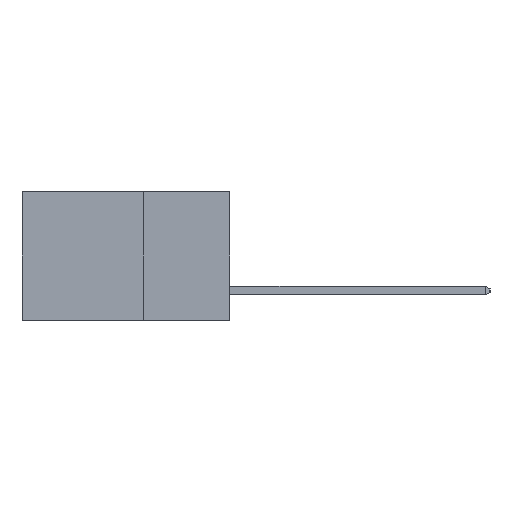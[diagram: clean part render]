
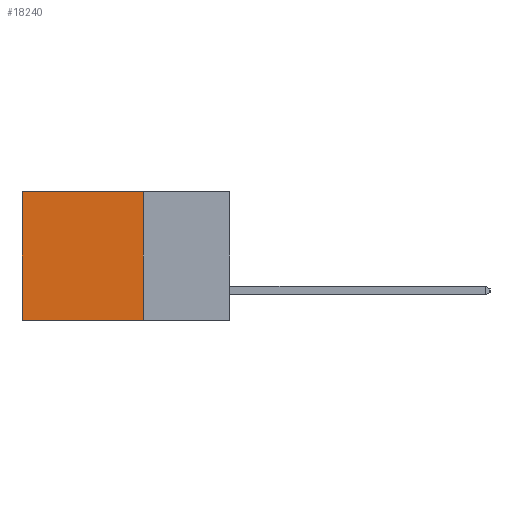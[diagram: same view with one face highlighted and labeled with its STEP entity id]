
A CAD part, left-side view. The second image highlights one B-rep face of the part: STEP entity #18240.
In plain terms, the highlighted planar face has unit normal (-1, 0, 0).
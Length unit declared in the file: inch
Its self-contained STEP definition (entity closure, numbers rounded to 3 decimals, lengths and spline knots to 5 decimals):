
#406 = VERTEX_POINT ( 'NONE', #3370 ) ;
#1237 = ORIENTED_EDGE ( 'NONE', *, *, #3281, .F. ) ;
#3281 = EDGE_CURVE ( 'NONE', #28011, #23730, #18194, .T. ) ;
#3370 = CARTESIAN_POINT ( 'NONE',  ( 0.298, 0.6, 0. ) ) ;
#4004 = CARTESIAN_POINT ( 'NONE',  ( 0.298, 0.6, -0.37 ) ) ;
#5310 = EDGE_CURVE ( 'NONE', #406, #12613, #32222, .T. ) ;
#5362 = VECTOR ( 'NONE', #13731, 39.37008 ) ;
#6385 = AXIS2_PLACEMENT_3D ( 'NONE', #22246, #7437, #24851 ) ;
#7437 = DIRECTION ( 'NONE',  ( 1., 0., 0. ) ) ;
#8690 = EDGE_LOOP ( 'NONE', ( #11857, #28076, #1237, #14813 ) ) ;
#8990 = CARTESIAN_POINT ( 'NONE',  ( 0.298, 0.6, 0. ) ) ;
#11723 = CARTESIAN_POINT ( 'NONE',  ( 0.298, 0.25, 0. ) ) ;
#11857 = ORIENTED_EDGE ( 'NONE', *, *, #5310, .T. ) ;
#12613 = VERTEX_POINT ( 'NONE', #4004 ) ;
#13731 = DIRECTION ( 'NONE',  ( 0., 1., 0. ) ) ;
#14813 = ORIENTED_EDGE ( 'NONE', *, *, #19359, .T. ) ;
#15311 = LINE ( 'NONE', #24009, #21906 ) ;
#17432 = VECTOR ( 'NONE', #25183, 39.37008 ) ;
#17674 = LINE ( 'NONE', #31253, #5362 ) ;
#18046 = VECTOR ( 'NONE', #29323, 39.37008 ) ;
#18194 = LINE ( 'NONE', #19132, #17432 ) ;
#18240 = ADVANCED_FACE ( 'NONE', ( #25203 ), #29758, .F. ) ;
#18876 = DIRECTION ( 'NONE',  ( 0., 1., 0. ) ) ;
#19132 = CARTESIAN_POINT ( 'NONE',  ( 0.298, 0.25, 0. ) ) ;
#19359 = EDGE_CURVE ( 'NONE', #28011, #406, #15311, .T. ) ;
#21906 = VECTOR ( 'NONE', #18876, 39.37008 ) ;
#22246 = CARTESIAN_POINT ( 'NONE',  ( 0.298, 0.25, 0. ) ) ;
#23730 = VERTEX_POINT ( 'NONE', #25295 ) ;
#24003 = EDGE_CURVE ( 'NONE', #23730, #12613, #17674, .T. ) ;
#24009 = CARTESIAN_POINT ( 'NONE',  ( 0.298, 0.25, 0. ) ) ;
#24851 = DIRECTION ( 'NONE',  ( 0., 0., -1. ) ) ;
#25183 = DIRECTION ( 'NONE',  ( 0., 0., -1. ) ) ;
#25203 = FACE_OUTER_BOUND ( 'NONE', #8690, .T. ) ;
#25295 = CARTESIAN_POINT ( 'NONE',  ( 0.298, 0.25, -0.37 ) ) ;
#28011 = VERTEX_POINT ( 'NONE', #11723 ) ;
#28076 = ORIENTED_EDGE ( 'NONE', *, *, #24003, .F. ) ;
#29323 = DIRECTION ( 'NONE',  ( 0., 0., -1. ) ) ;
#29758 = PLANE ( 'NONE',  #6385 ) ;
#31253 = CARTESIAN_POINT ( 'NONE',  ( 0.298, 0.25, -0.37 ) ) ;
#32222 = LINE ( 'NONE', #8990, #18046 ) ;
